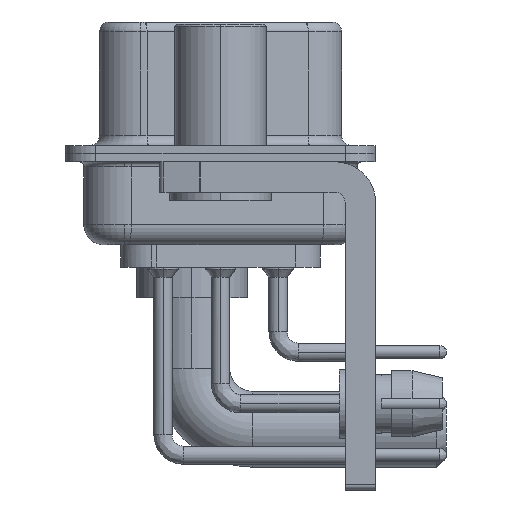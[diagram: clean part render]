
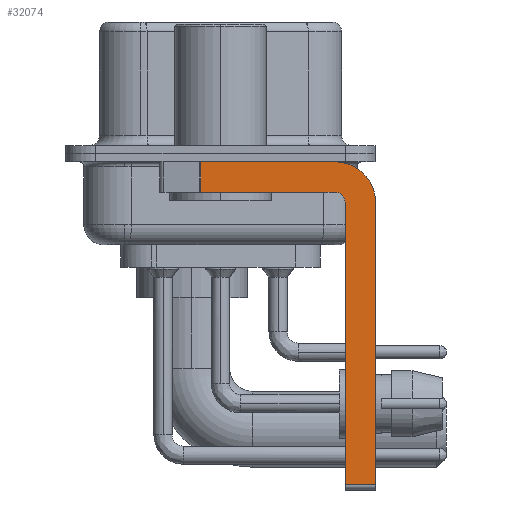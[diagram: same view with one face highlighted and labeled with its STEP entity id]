
A CAD part, left-side view. The second image highlights one B-rep face of the part: STEP entity #32074.
In plain terms, the highlighted planar face has unit normal (-1, 0, 0).
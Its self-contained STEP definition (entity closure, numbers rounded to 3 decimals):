
#545 = DIRECTION ( 'NONE',  ( 0., 1., 0. ) ) ;
#1122 = DIRECTION ( 'NONE',  ( 0., 0., -1. ) ) ;
#1613 = VERTEX_POINT ( 'NONE', #5554 ) ;
#1758 = DIRECTION ( 'NONE',  ( 0., -1., 0. ) ) ;
#2290 = EDGE_CURVE ( 'NONE', #1613, #29574, #8265, .T. ) ;
#2516 = PLANE ( 'NONE',  #29472 ) ;
#2903 = CIRCLE ( 'NONE', #28985, 2. ) ;
#3444 = VERTEX_POINT ( 'NONE', #8991 ) ;
#3760 = DIRECTION ( 'NONE',  ( -1., 0., 0. ) ) ;
#4004 = ORIENTED_EDGE ( 'NONE', *, *, #2290, .T. ) ;
#5554 = CARTESIAN_POINT ( 'NONE',  ( -2.9, -6.15, -16.35 ) ) ;
#6803 = VECTOR ( 'NONE', #29590, 1000. ) ;
#6954 = VECTOR ( 'NONE', #39303, 1000. ) ;
#7208 = DIRECTION ( 'NONE',  ( 0., 0., -1. ) ) ;
#7850 = CARTESIAN_POINT ( 'NONE',  ( -2.9, -7.65, -2.4 ) ) ;
#8265 = LINE ( 'NONE', #23382, #12081 ) ;
#8429 = EDGE_LOOP ( 'NONE', ( #39591, #21485, #19297, #38178, #31142, #4004, #34896, #26532 ) ) ;
#8840 = DIRECTION ( 'NONE',  ( 1., 0., 0. ) ) ;
#8894 = CARTESIAN_POINT ( 'NONE',  ( -2.9, -5.65, -0.4 ) ) ;
#8991 = CARTESIAN_POINT ( 'NONE',  ( -2.9, -5.65, -1.9 ) ) ;
#9862 = VECTOR ( 'NONE', #545, 1000. ) ;
#10431 = VERTEX_POINT ( 'NONE', #8894 ) ;
#10702 = EDGE_CURVE ( 'NONE', #10431, #20424, #2903, .T. ) ;
#11085 = CARTESIAN_POINT ( 'NONE',  ( -2.9, -5.65, -2.4 ) ) ;
#12081 = VECTOR ( 'NONE', #1758, 1000. ) ;
#12599 = CARTESIAN_POINT ( 'NONE',  ( -2.9, 0.978, -0.4 ) ) ;
#13435 = VECTOR ( 'NONE', #7208, 1000. ) ;
#15145 = VERTEX_POINT ( 'NONE', #12599 ) ;
#16291 = VERTEX_POINT ( 'NONE', #33073 ) ;
#16573 = LINE ( 'NONE', #32130, #13435 ) ;
#17390 = DIRECTION ( 'NONE',  ( 0., 0., -1. ) ) ;
#18001 = FACE_OUTER_BOUND ( 'NONE', #8429, .T. ) ;
#18878 = LINE ( 'NONE', #37916, #9862 ) ;
#19297 = ORIENTED_EDGE ( 'NONE', *, *, #29469, .F. ) ;
#19374 = LINE ( 'NONE', #35136, #6803 ) ;
#19654 = DIRECTION ( 'NONE',  ( 1., 0., 0. ) ) ;
#20424 = VERTEX_POINT ( 'NONE', #23079 ) ;
#21354 = EDGE_CURVE ( 'NONE', #15145, #37533, #16573, .T. ) ;
#21485 = ORIENTED_EDGE ( 'NONE', *, *, #21354, .T. ) ;
#22734 = CARTESIAN_POINT ( 'NONE',  ( -2.9, 0.978, -1.9 ) ) ;
#23079 = CARTESIAN_POINT ( 'NONE',  ( -2.9, -7.65, -2.4 ) ) ;
#23382 = CARTESIAN_POINT ( 'NONE',  ( -2.9, -5.65, -16.35 ) ) ;
#23473 = EDGE_CURVE ( 'NONE', #20424, #29574, #24170, .T. ) ;
#24170 = LINE ( 'NONE', #7850, #6954 ) ;
#24351 = VECTOR ( 'NONE', #25252, 1000. ) ;
#25252 = DIRECTION ( 'NONE',  ( 0., 0., 1. ) ) ;
#26493 = CIRCLE ( 'NONE', #30406, 0.5 ) ;
#26532 = ORIENTED_EDGE ( 'NONE', *, *, #10702, .F. ) ;
#28657 = DIRECTION ( 'NONE',  ( 0., 0., 1. ) ) ;
#28985 = AXIS2_PLACEMENT_3D ( 'NONE', #11085, #19654, #1122 ) ;
#29469 = EDGE_CURVE ( 'NONE', #3444, #37533, #18878, .T. ) ;
#29472 = AXIS2_PLACEMENT_3D ( 'NONE', #36827, #8840, #17390 ) ;
#29574 = VERTEX_POINT ( 'NONE', #36044 ) ;
#29590 = DIRECTION ( 'NONE',  ( 0., -1., 0. ) ) ;
#30406 = AXIS2_PLACEMENT_3D ( 'NONE', #35201, #3760, #28657 ) ;
#31142 = ORIENTED_EDGE ( 'NONE', *, *, #38807, .F. ) ;
#32074 = ADVANCED_FACE ( 'NONE', ( #18001 ), #2516, .F. ) ;
#32130 = CARTESIAN_POINT ( 'NONE',  ( -2.9, 0.978, -1.9 ) ) ;
#33073 = CARTESIAN_POINT ( 'NONE',  ( -2.9, -6.15, -2.4 ) ) ;
#34158 = EDGE_CURVE ( 'NONE', #15145, #10431, #19374, .T. ) ;
#34896 = ORIENTED_EDGE ( 'NONE', *, *, #23473, .F. ) ;
#35068 = LINE ( 'NONE', #38329, #24351 ) ;
#35136 = CARTESIAN_POINT ( 'NONE',  ( -2.9, 3., -0.4 ) ) ;
#35201 = CARTESIAN_POINT ( 'NONE',  ( -2.9, -5.65, -2.4 ) ) ;
#36044 = CARTESIAN_POINT ( 'NONE',  ( -2.9, -7.65, -16.35 ) ) ;
#36827 = CARTESIAN_POINT ( 'NONE',  ( -2.9, -5.65, -2.4 ) ) ;
#37533 = VERTEX_POINT ( 'NONE', #22734 ) ;
#37535 = EDGE_CURVE ( 'NONE', #16291, #3444, #26493, .T. ) ;
#37916 = CARTESIAN_POINT ( 'NONE',  ( -2.9, -5.65, -1.9 ) ) ;
#38178 = ORIENTED_EDGE ( 'NONE', *, *, #37535, .F. ) ;
#38329 = CARTESIAN_POINT ( 'NONE',  ( -2.9, -6.15, -16.6 ) ) ;
#38807 = EDGE_CURVE ( 'NONE', #1613, #16291, #35068, .T. ) ;
#39303 = DIRECTION ( 'NONE',  ( 0., 0., -1. ) ) ;
#39591 = ORIENTED_EDGE ( 'NONE', *, *, #34158, .F. ) ;
